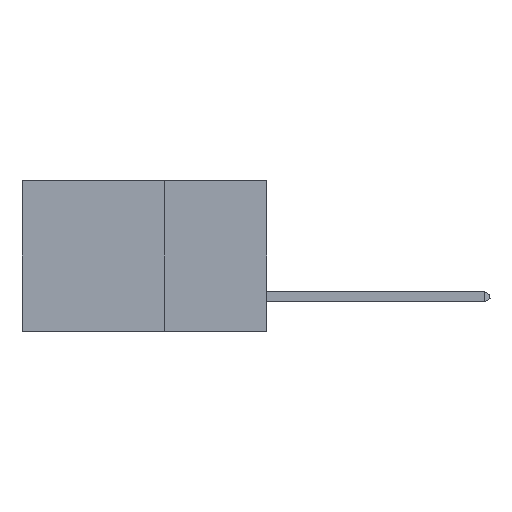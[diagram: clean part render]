
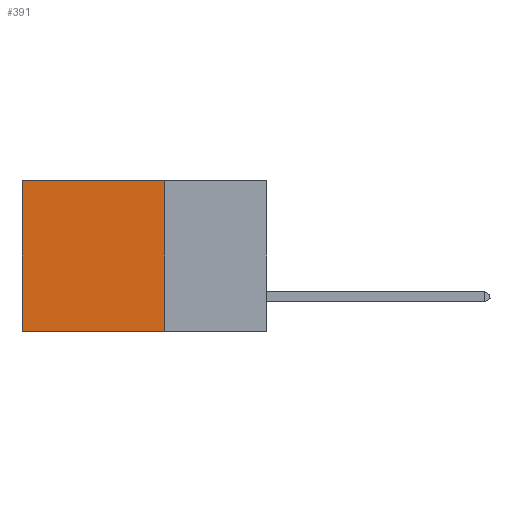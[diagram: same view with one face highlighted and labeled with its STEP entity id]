
A CAD part, left-side view. The second image highlights one B-rep face of the part: STEP entity #391.
In plain terms, the highlighted planar face has unit normal (-1, 0, 0).
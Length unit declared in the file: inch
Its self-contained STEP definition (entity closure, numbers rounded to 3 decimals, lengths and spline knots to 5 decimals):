
#162 = CARTESIAN_POINT ( 'NONE',  ( 0.2875, 0.25, -0.37 ) ) ;
#250 = ORIENTED_EDGE ( 'NONE', *, *, #2149, .F. ) ;
#391 = ADVANCED_FACE ( 'NONE', ( #13116 ), #16448, .F. ) ;
#470 = AXIS2_PLACEMENT_3D ( 'NONE', #14877, #17892, #8903 ) ;
#1928 = CARTESIAN_POINT ( 'NONE',  ( 0.2875, 0.6, 0. ) ) ;
#2149 = EDGE_CURVE ( 'NONE', #17990, #8302, #16014, .T. ) ;
#2910 = VECTOR ( 'NONE', #16463, 39.37008 ) ;
#3405 = EDGE_CURVE ( 'NONE', #10021, #5573, #12933, .T. ) ;
#3641 = CARTESIAN_POINT ( 'NONE',  ( 0.2875, 0.6, -0.37 ) ) ;
#4109 = LINE ( 'NONE', #7608, #8812 ) ;
#4458 = CARTESIAN_POINT ( 'NONE',  ( 0.2875, 0.25, 0. ) ) ;
#5076 = ORIENTED_EDGE ( 'NONE', *, *, #3405, .T. ) ;
#5573 = VERTEX_POINT ( 'NONE', #3641 ) ;
#5840 = LINE ( 'NONE', #7404, #12855 ) ;
#6225 = DIRECTION ( 'NONE',  ( 0., 0., -1. ) ) ;
#7143 = DIRECTION ( 'NONE',  ( 0., 1., 0. ) ) ;
#7404 = CARTESIAN_POINT ( 'NONE',  ( 0.2875, 0.25, 0. ) ) ;
#7608 = CARTESIAN_POINT ( 'NONE',  ( 0.2875, 0.25, -0.37 ) ) ;
#8302 = VERTEX_POINT ( 'NONE', #162 ) ;
#8812 = VECTOR ( 'NONE', #12375, 39.37008 ) ;
#8903 = DIRECTION ( 'NONE',  ( 0., 0., -1. ) ) ;
#10021 = VERTEX_POINT ( 'NONE', #1928 ) ;
#11452 = EDGE_CURVE ( 'NONE', #8302, #5573, #4109, .T. ) ;
#12375 = DIRECTION ( 'NONE',  ( 0., 1., 0. ) ) ;
#12855 = VECTOR ( 'NONE', #7143, 39.37008 ) ;
#12933 = LINE ( 'NONE', #16741, #15748 ) ;
#13116 = FACE_OUTER_BOUND ( 'NONE', #18681, .T. ) ;
#14552 = CARTESIAN_POINT ( 'NONE',  ( 0.2875, 0.25, 0. ) ) ;
#14877 = CARTESIAN_POINT ( 'NONE',  ( 0.2875, 0.25, 0. ) ) ;
#15748 = VECTOR ( 'NONE', #6225, 39.37008 ) ;
#16014 = LINE ( 'NONE', #4458, #2910 ) ;
#16178 = EDGE_CURVE ( 'NONE', #17990, #10021, #5840, .T. ) ;
#16239 = ORIENTED_EDGE ( 'NONE', *, *, #16178, .T. ) ;
#16448 = PLANE ( 'NONE',  #470 ) ;
#16463 = DIRECTION ( 'NONE',  ( 0., 0., -1. ) ) ;
#16741 = CARTESIAN_POINT ( 'NONE',  ( 0.2875, 0.6, 0. ) ) ;
#17593 = ORIENTED_EDGE ( 'NONE', *, *, #11452, .F. ) ;
#17892 = DIRECTION ( 'NONE',  ( 1., 0., 0. ) ) ;
#17990 = VERTEX_POINT ( 'NONE', #14552 ) ;
#18681 = EDGE_LOOP ( 'NONE', ( #5076, #17593, #250, #16239 ) ) ;
